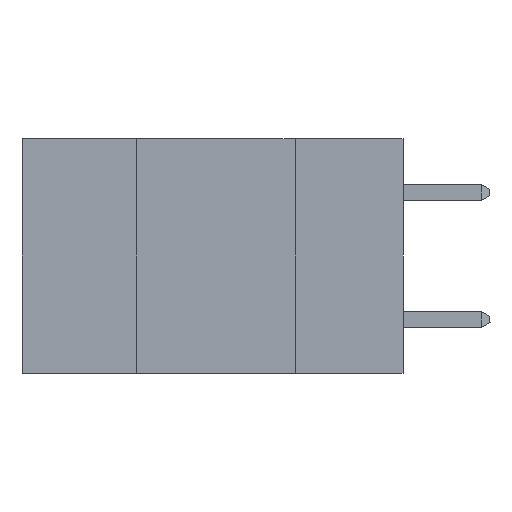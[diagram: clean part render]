
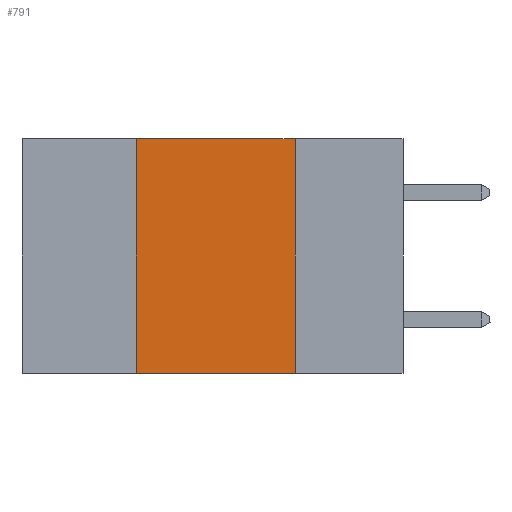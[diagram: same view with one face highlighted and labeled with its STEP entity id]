
A CAD part, left-side view. The second image highlights one B-rep face of the part: STEP entity #791.
In plain terms, the highlighted planar face has unit normal (-1, 0, 0).
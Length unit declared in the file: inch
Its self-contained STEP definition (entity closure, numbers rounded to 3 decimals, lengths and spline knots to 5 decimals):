
#791 = ADVANCED_FACE ( 'NONE', ( #11108 ), #15166, .F. ) ;
#1296 = CARTESIAN_POINT ( 'NONE',  ( 0., 0.42, 0. ) ) ;
#1327 = VERTEX_POINT ( 'NONE', #16041 ) ;
#1858 = CARTESIAN_POINT ( 'NONE',  ( 0., 0.17, 0. ) ) ;
#3019 = VERTEX_POINT ( 'NONE', #5914 ) ;
#3403 = DIRECTION ( 'NONE',  ( 1., 0., 0. ) ) ;
#4153 = DIRECTION ( 'NONE',  ( 0., -1., 0. ) ) ;
#4714 = ORIENTED_EDGE ( 'NONE', *, *, #10392, .F. ) ;
#5059 = VERTEX_POINT ( 'NONE', #11519 ) ;
#5888 = CARTESIAN_POINT ( 'NONE',  ( 0., 0.6, -0.37 ) ) ;
#5914 = CARTESIAN_POINT ( 'NONE',  ( 0., 0.17, 0. ) ) ;
#6416 = CARTESIAN_POINT ( 'NONE',  ( 0., 0.42, 0. ) ) ;
#8469 = VECTOR ( 'NONE', #22420, 39.37008 ) ;
#8855 = VECTOR ( 'NONE', #23869, 39.37008 ) ;
#9335 = CARTESIAN_POINT ( 'NONE',  ( 0., 0.6, 0. ) ) ;
#9738 = EDGE_CURVE ( 'NONE', #21957, #3019, #13908, .T. ) ;
#10000 = ORIENTED_EDGE ( 'NONE', *, *, #9738, .F. ) ;
#10164 = CARTESIAN_POINT ( 'NONE',  ( 0., 0.6, 0. ) ) ;
#10392 = EDGE_CURVE ( 'NONE', #3019, #5059, #13545, .T. ) ;
#11108 = FACE_OUTER_BOUND ( 'NONE', #12707, .T. ) ;
#11519 = CARTESIAN_POINT ( 'NONE',  ( 0., 0.17, -0.37 ) ) ;
#12128 = EDGE_CURVE ( 'NONE', #1327, #21957, #20989, .T. ) ;
#12661 = VECTOR ( 'NONE', #4153, 39.37008 ) ;
#12707 = EDGE_LOOP ( 'NONE', ( #4714, #10000, #19640, #24305 ) ) ;
#13545 = LINE ( 'NONE', #1858, #8855 ) ;
#13908 = LINE ( 'NONE', #10164, #12661 ) ;
#15021 = DIRECTION ( 'NONE',  ( 0., 0., -1. ) ) ;
#15166 = PLANE ( 'NONE',  #20657 ) ;
#16041 = CARTESIAN_POINT ( 'NONE',  ( 0., 0.42, -0.37 ) ) ;
#16650 = EDGE_CURVE ( 'NONE', #1327, #5059, #25346, .T. ) ;
#19640 = ORIENTED_EDGE ( 'NONE', *, *, #12128, .F. ) ;
#20176 = VECTOR ( 'NONE', #21918, 39.37008 ) ;
#20657 = AXIS2_PLACEMENT_3D ( 'NONE', #9335, #3403, #15021 ) ;
#20989 = LINE ( 'NONE', #6416, #8469 ) ;
#21918 = DIRECTION ( 'NONE',  ( 0., -1., 0. ) ) ;
#21957 = VERTEX_POINT ( 'NONE', #1296 ) ;
#22420 = DIRECTION ( 'NONE',  ( 0., 0., 1. ) ) ;
#23869 = DIRECTION ( 'NONE',  ( 0., 0., -1. ) ) ;
#24305 = ORIENTED_EDGE ( 'NONE', *, *, #16650, .T. ) ;
#25346 = LINE ( 'NONE', #5888, #20176 ) ;
